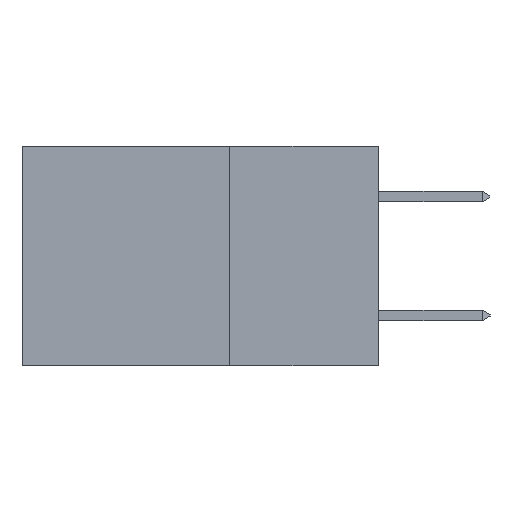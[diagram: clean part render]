
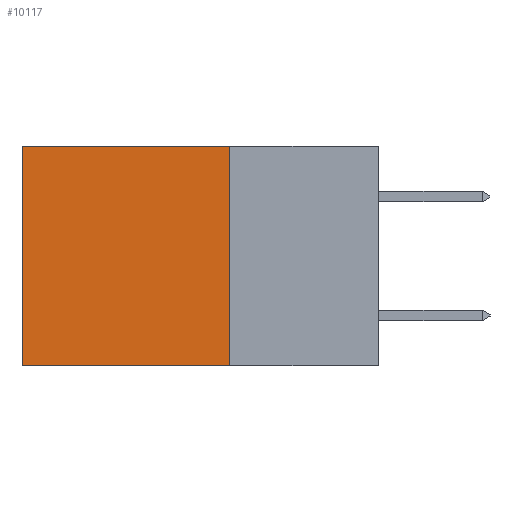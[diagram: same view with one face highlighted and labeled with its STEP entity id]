
A CAD part, left-side view. The second image highlights one B-rep face of the part: STEP entity #10117.
In plain terms, the highlighted planar face has unit normal (-1, 0, 0).
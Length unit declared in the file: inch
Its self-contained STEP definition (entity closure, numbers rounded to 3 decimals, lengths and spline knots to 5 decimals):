
#199 = LINE ( 'NONE', #7953, #2858 ) ;
#486 = EDGE_CURVE ( 'NONE', #1280, #2722, #12260, .T. ) ;
#795 = LINE ( 'NONE', #8900, #3340 ) ;
#1100 = DIRECTION ( 'NONE',  ( 1., 0., 0. ) ) ;
#1147 = VERTEX_POINT ( 'NONE', #8862 ) ;
#1280 = VERTEX_POINT ( 'NONE', #4012 ) ;
#1565 = EDGE_CURVE ( 'NONE', #1280, #1147, #199, .T. ) ;
#1612 = ORIENTED_EDGE ( 'NONE', *, *, #486, .F. ) ;
#1848 = EDGE_LOOP ( 'NONE', ( #10079, #11438, #1612, #11321 ) ) ;
#1984 = EDGE_CURVE ( 'NONE', #1147, #5093, #10650, .T. ) ;
#2722 = VERTEX_POINT ( 'NONE', #7513 ) ;
#2858 = VECTOR ( 'NONE', #7532, 39.37008 ) ;
#3301 = DIRECTION ( 'NONE',  ( 0., 0., -1. ) ) ;
#3340 = VECTOR ( 'NONE', #14197, 39.37008 ) ;
#3616 = VECTOR ( 'NONE', #3666, 39.37008 ) ;
#3666 = DIRECTION ( 'NONE',  ( 0., 0., -1. ) ) ;
#3723 = CARTESIAN_POINT ( 'NONE',  ( 0.2615, 0.6, -0.37 ) ) ;
#4012 = CARTESIAN_POINT ( 'NONE',  ( 0.2615, 0.25, 0. ) ) ;
#4542 = FACE_OUTER_BOUND ( 'NONE', #1848, .T. ) ;
#4941 = CARTESIAN_POINT ( 'NONE',  ( 0.2615, 0.25, -0.37 ) ) ;
#5093 = VERTEX_POINT ( 'NONE', #8977 ) ;
#6862 = CARTESIAN_POINT ( 'NONE',  ( 0.2615, 0.25, -0.37 ) ) ;
#7496 = VECTOR ( 'NONE', #3301, 39.37008 ) ;
#7513 = CARTESIAN_POINT ( 'NONE',  ( 0.2615, 0.25, -0.37 ) ) ;
#7532 = DIRECTION ( 'NONE',  ( 0., 1., 0. ) ) ;
#7953 = CARTESIAN_POINT ( 'NONE',  ( 0.2615, 0.25, 0. ) ) ;
#8862 = CARTESIAN_POINT ( 'NONE',  ( 0.2615, 0.6, 0. ) ) ;
#8900 = CARTESIAN_POINT ( 'NONE',  ( 0.2615, 0.25, -0.37 ) ) ;
#8977 = CARTESIAN_POINT ( 'NONE',  ( 0.2615, 0.6, -0.37 ) ) ;
#9001 = DIRECTION ( 'NONE',  ( 0., 0., -1. ) ) ;
#9430 = AXIS2_PLACEMENT_3D ( 'NONE', #6862, #1100, #9001 ) ;
#10079 = ORIENTED_EDGE ( 'NONE', *, *, #1984, .T. ) ;
#10117 = ADVANCED_FACE ( 'NONE', ( #4542 ), #13270, .F. ) ;
#10650 = LINE ( 'NONE', #3723, #7496 ) ;
#11321 = ORIENTED_EDGE ( 'NONE', *, *, #1565, .T. ) ;
#11438 = ORIENTED_EDGE ( 'NONE', *, *, #13042, .F. ) ;
#12260 = LINE ( 'NONE', #4941, #3616 ) ;
#13042 = EDGE_CURVE ( 'NONE', #2722, #5093, #795, .T. ) ;
#13270 = PLANE ( 'NONE',  #9430 ) ;
#14197 = DIRECTION ( 'NONE',  ( 0., 1., 0. ) ) ;
